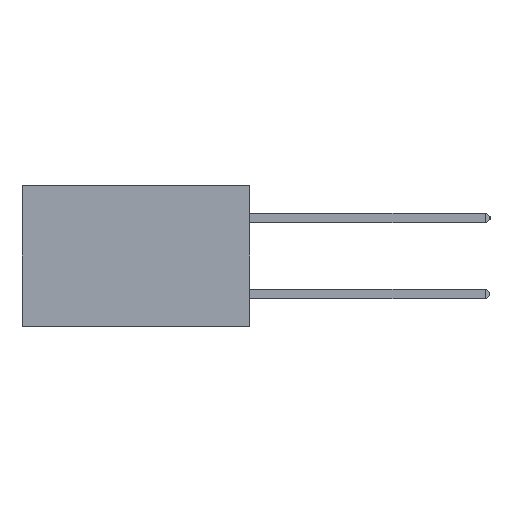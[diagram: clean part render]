
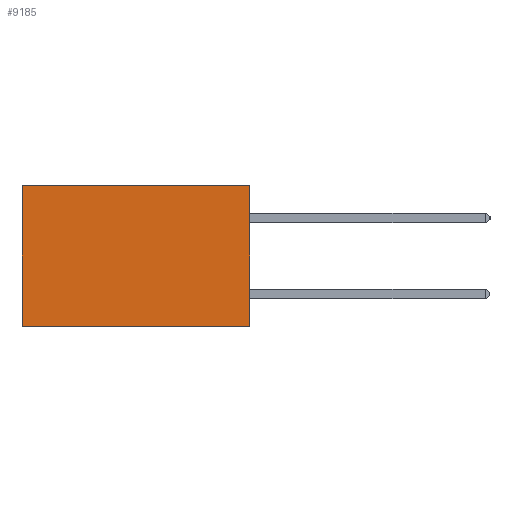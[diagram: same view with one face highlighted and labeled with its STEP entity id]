
A CAD part, left-side view. The second image highlights one B-rep face of the part: STEP entity #9185.
In plain terms, the highlighted planar face has unit normal (-1, 0, 0).
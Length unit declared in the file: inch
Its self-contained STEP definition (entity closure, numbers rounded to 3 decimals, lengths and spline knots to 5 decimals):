
#1021 = PLANE ( 'NONE',  #2431 ) ;
#1403 = DIRECTION ( 'NONE',  ( 0., 1., 0. ) ) ;
#2143 = CARTESIAN_POINT ( 'NONE',  ( 0.2875, 0.6, -0.37 ) ) ;
#2431 = AXIS2_PLACEMENT_3D ( 'NONE', #21071, #4387, #16148 ) ;
#3948 = EDGE_CURVE ( 'NONE', #19700, #19658, #7211, .T. ) ;
#3965 = CARTESIAN_POINT ( 'NONE',  ( 0.2875, 0., 0. ) ) ;
#4294 = DIRECTION ( 'NONE',  ( 0., 0., -1. ) ) ;
#4387 = DIRECTION ( 'NONE',  ( 1., 0., 0. ) ) ;
#4523 = LINE ( 'NONE', #13071, #9525 ) ;
#4796 = EDGE_CURVE ( 'NONE', #10923, #20799, #13141, .T. ) ;
#5655 = ORIENTED_EDGE ( 'NONE', *, *, #21602, .T. ) ;
#5673 = DIRECTION ( 'NONE',  ( 0., 1., 0. ) ) ;
#5969 = VECTOR ( 'NONE', #5673, 39.37008 ) ;
#7211 = LINE ( 'NONE', #14293, #20577 ) ;
#8228 = VECTOR ( 'NONE', #10000, 39.37008 ) ;
#9185 = ADVANCED_FACE ( 'NONE', ( #12880 ), #1021, .F. ) ;
#9525 = VECTOR ( 'NONE', #1403, 39.37008 ) ;
#10000 = DIRECTION ( 'NONE',  ( 0., 0., -1. ) ) ;
#10923 = VERTEX_POINT ( 'NONE', #20964 ) ;
#10960 = EDGE_LOOP ( 'NONE', ( #12929, #15116, #15602, #5655 ) ) ;
#12454 = CARTESIAN_POINT ( 'NONE',  ( 0.2875, 0., -0.37 ) ) ;
#12880 = FACE_OUTER_BOUND ( 'NONE', #10960, .T. ) ;
#12929 = ORIENTED_EDGE ( 'NONE', *, *, #4796, .T. ) ;
#13071 = CARTESIAN_POINT ( 'NONE',  ( 0.2875, 0., -0.37 ) ) ;
#13141 = LINE ( 'NONE', #14970, #8228 ) ;
#14293 = CARTESIAN_POINT ( 'NONE',  ( 0.2875, 0., 0. ) ) ;
#14869 = LINE ( 'NONE', #3965, #5969 ) ;
#14970 = CARTESIAN_POINT ( 'NONE',  ( 0.2875, 0.6, 0. ) ) ;
#15116 = ORIENTED_EDGE ( 'NONE', *, *, #16265, .F. ) ;
#15602 = ORIENTED_EDGE ( 'NONE', *, *, #3948, .F. ) ;
#16148 = DIRECTION ( 'NONE',  ( 0., 0., -1. ) ) ;
#16265 = EDGE_CURVE ( 'NONE', #19658, #20799, #4523, .T. ) ;
#17741 = CARTESIAN_POINT ( 'NONE',  ( 0.2875, 0., 0. ) ) ;
#19658 = VERTEX_POINT ( 'NONE', #12454 ) ;
#19700 = VERTEX_POINT ( 'NONE', #17741 ) ;
#20577 = VECTOR ( 'NONE', #4294, 39.37008 ) ;
#20799 = VERTEX_POINT ( 'NONE', #2143 ) ;
#20964 = CARTESIAN_POINT ( 'NONE',  ( 0.2875, 0.6, 0. ) ) ;
#21071 = CARTESIAN_POINT ( 'NONE',  ( 0.2875, 0., 0. ) ) ;
#21602 = EDGE_CURVE ( 'NONE', #19700, #10923, #14869, .T. ) ;
